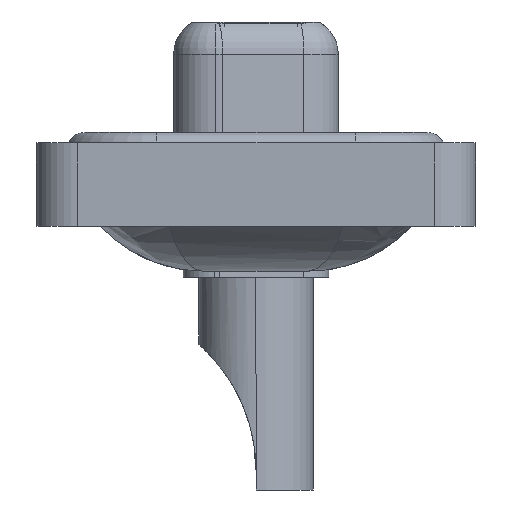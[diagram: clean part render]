
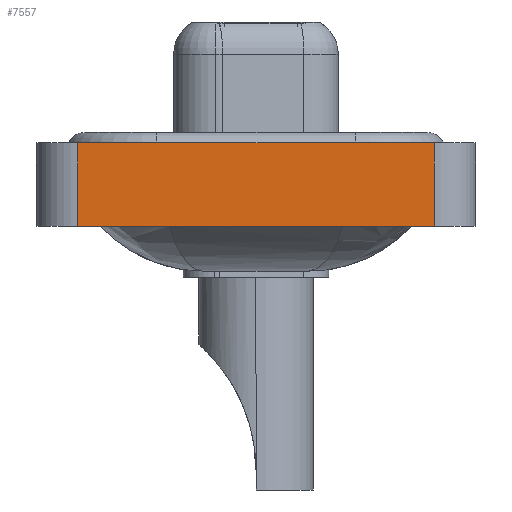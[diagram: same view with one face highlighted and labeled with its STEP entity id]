
A CAD part, left-side view. The second image highlights one B-rep face of the part: STEP entity #7557.
In plain terms, the highlighted planar face has unit normal (-1, 0, 0).
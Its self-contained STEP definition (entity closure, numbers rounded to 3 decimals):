
#1299 = CARTESIAN_POINT ( 'NONE',  ( -7.35, 8.55, -3.6 ) ) ;
#1714 = VECTOR ( 'NONE', #3447, 1000. ) ;
#1955 = LINE ( 'NONE', #13296, #7579 ) ;
#2047 = EDGE_CURVE ( 'NONE', #11751, #5597, #15014, .T. ) ;
#2990 = CARTESIAN_POINT ( 'NONE',  ( -7.35, -8.55, -3.6 ) ) ;
#3447 = DIRECTION ( 'NONE',  ( 0., -1., 0. ) ) ;
#4118 = PLANE ( 'NONE',  #8171 ) ;
#4843 = ORIENTED_EDGE ( 'NONE', *, *, #8434, .T. ) ;
#5597 = VERTEX_POINT ( 'NONE', #18381 ) ;
#5700 = FACE_OUTER_BOUND ( 'NONE', #17618, .T. ) ;
#7255 = CARTESIAN_POINT ( 'NONE',  ( -7.35, -8.55, -3.6 ) ) ;
#7557 = ADVANCED_FACE ( 'NONE', ( #5700 ), #4118, .T. ) ;
#7579 = VECTOR ( 'NONE', #13187, 1000. ) ;
#7748 = EDGE_CURVE ( 'NONE', #10399, #11751, #9412, .T. ) ;
#8171 = AXIS2_PLACEMENT_3D ( 'NONE', #10590, #11971, #18477 ) ;
#8207 = VECTOR ( 'NONE', #13696, 1000. ) ;
#8434 = EDGE_CURVE ( 'NONE', #10399, #12621, #12098, .T. ) ;
#8847 = VECTOR ( 'NONE', #16002, 1000. ) ;
#9212 = CARTESIAN_POINT ( 'NONE',  ( -7.35, 8.55, -3.6 ) ) ;
#9412 = LINE ( 'NONE', #9212, #8847 ) ;
#10399 = VERTEX_POINT ( 'NONE', #1299 ) ;
#10590 = CARTESIAN_POINT ( 'NONE',  ( -7.35, -8.55, -3.6 ) ) ;
#11751 = VERTEX_POINT ( 'NONE', #18689 ) ;
#11971 = DIRECTION ( 'NONE',  ( -1., 0., 0. ) ) ;
#12098 = LINE ( 'NONE', #7255, #8207 ) ;
#12621 = VERTEX_POINT ( 'NONE', #2990 ) ;
#13187 = DIRECTION ( 'NONE',  ( 0., 0., 1. ) ) ;
#13296 = CARTESIAN_POINT ( 'NONE',  ( -7.35, -8.55, -3.6 ) ) ;
#13310 = CARTESIAN_POINT ( 'NONE',  ( -7.35, -8.55, 0.4 ) ) ;
#13696 = DIRECTION ( 'NONE',  ( 0., -1., 0. ) ) ;
#15014 = LINE ( 'NONE', #13310, #1714 ) ;
#16002 = DIRECTION ( 'NONE',  ( 0., 0., 1. ) ) ;
#16040 = ORIENTED_EDGE ( 'NONE', *, *, #17626, .T. ) ;
#16927 = ORIENTED_EDGE ( 'NONE', *, *, #2047, .F. ) ;
#17618 = EDGE_LOOP ( 'NONE', ( #16040, #16927, #18987, #4843 ) ) ;
#17626 = EDGE_CURVE ( 'NONE', #12621, #5597, #1955, .T. ) ;
#18381 = CARTESIAN_POINT ( 'NONE',  ( -7.35, -8.55, 0.4 ) ) ;
#18477 = DIRECTION ( 'NONE',  ( 0., 0., 1. ) ) ;
#18689 = CARTESIAN_POINT ( 'NONE',  ( -7.35, 8.55, 0.4 ) ) ;
#18987 = ORIENTED_EDGE ( 'NONE', *, *, #7748, .F. ) ;
